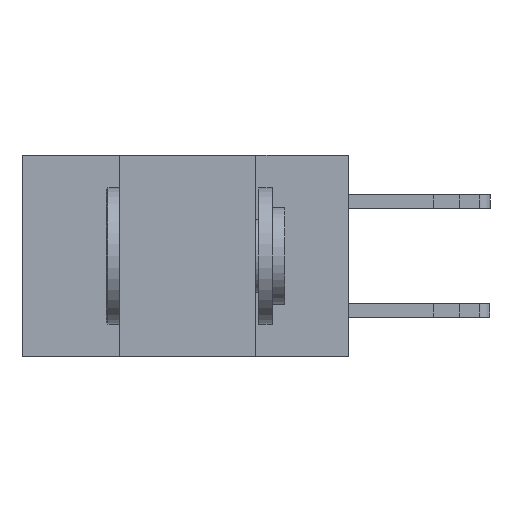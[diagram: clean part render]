
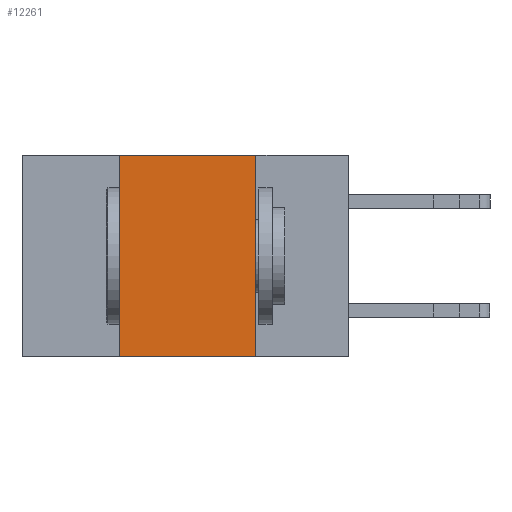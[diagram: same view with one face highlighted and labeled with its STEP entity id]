
A CAD part, left-side view. The second image highlights one B-rep face of the part: STEP entity #12261.
In plain terms, the highlighted planar face has unit normal (-1, 0, 0).
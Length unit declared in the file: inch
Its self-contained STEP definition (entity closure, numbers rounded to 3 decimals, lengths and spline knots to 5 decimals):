
#445 = LINE ( 'NONE', #9860, #6425 ) ;
#1478 = EDGE_CURVE ( 'NONE', #6712, #11704, #445, .T. ) ;
#1547 = DIRECTION ( 'NONE',  ( 0., -1., 0. ) ) ;
#2142 = LINE ( 'NONE', #5084, #14276 ) ;
#2227 = CARTESIAN_POINT ( 'NONE',  ( 0., 0.17, 0. ) ) ;
#2853 = CARTESIAN_POINT ( 'NONE',  ( 0., 0.17, 0. ) ) ;
#3884 = CARTESIAN_POINT ( 'NONE',  ( 0., 0.6, 0. ) ) ;
#4083 = DIRECTION ( 'NONE',  ( 0., 0., -1. ) ) ;
#4588 = VECTOR ( 'NONE', #9075, 39.37008 ) ;
#4708 = DIRECTION ( 'NONE',  ( 0., -1., 0. ) ) ;
#5046 = DIRECTION ( 'NONE',  ( 0., 0., -1. ) ) ;
#5084 = CARTESIAN_POINT ( 'NONE',  ( 0., 0.6, -0.37 ) ) ;
#5559 = VECTOR ( 'NONE', #4083, 39.37008 ) ;
#5846 = AXIS2_PLACEMENT_3D ( 'NONE', #3884, #12078, #5046 ) ;
#6425 = VECTOR ( 'NONE', #1547, 39.37008 ) ;
#6712 = VERTEX_POINT ( 'NONE', #13980 ) ;
#6714 = VERTEX_POINT ( 'NONE', #6795 ) ;
#6795 = CARTESIAN_POINT ( 'NONE',  ( 0., 0.17, -0.37 ) ) ;
#7314 = ORIENTED_EDGE ( 'NONE', *, *, #1478, .F. ) ;
#7371 = ORIENTED_EDGE ( 'NONE', *, *, #12364, .F. ) ;
#8923 = EDGE_CURVE ( 'NONE', #10162, #6714, #2142, .T. ) ;
#9075 = DIRECTION ( 'NONE',  ( 0., 0., 1. ) ) ;
#9101 = CARTESIAN_POINT ( 'NONE',  ( 0., 0.42, 0. ) ) ;
#9176 = EDGE_LOOP ( 'NONE', ( #7371, #7314, #11412, #12011 ) ) ;
#9423 = EDGE_CURVE ( 'NONE', #10162, #6712, #11542, .T. ) ;
#9781 = FACE_OUTER_BOUND ( 'NONE', #9176, .T. ) ;
#9860 = CARTESIAN_POINT ( 'NONE',  ( 0., 0.6, 0. ) ) ;
#10162 = VERTEX_POINT ( 'NONE', #13452 ) ;
#10896 = PLANE ( 'NONE',  #5846 ) ;
#11412 = ORIENTED_EDGE ( 'NONE', *, *, #9423, .F. ) ;
#11437 = LINE ( 'NONE', #2853, #5559 ) ;
#11542 = LINE ( 'NONE', #9101, #4588 ) ;
#11704 = VERTEX_POINT ( 'NONE', #2227 ) ;
#12011 = ORIENTED_EDGE ( 'NONE', *, *, #8923, .T. ) ;
#12078 = DIRECTION ( 'NONE',  ( 1., 0., 0. ) ) ;
#12261 = ADVANCED_FACE ( 'NONE', ( #9781 ), #10896, .F. ) ;
#12364 = EDGE_CURVE ( 'NONE', #11704, #6714, #11437, .T. ) ;
#13452 = CARTESIAN_POINT ( 'NONE',  ( 0., 0.42, -0.37 ) ) ;
#13980 = CARTESIAN_POINT ( 'NONE',  ( 0., 0.42, 0. ) ) ;
#14276 = VECTOR ( 'NONE', #4708, 39.37008 ) ;
